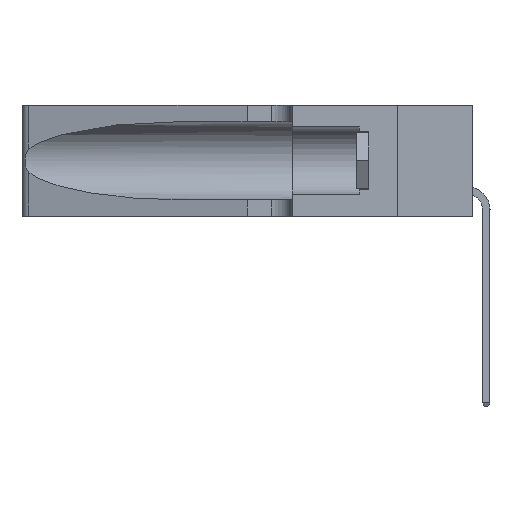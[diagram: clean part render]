
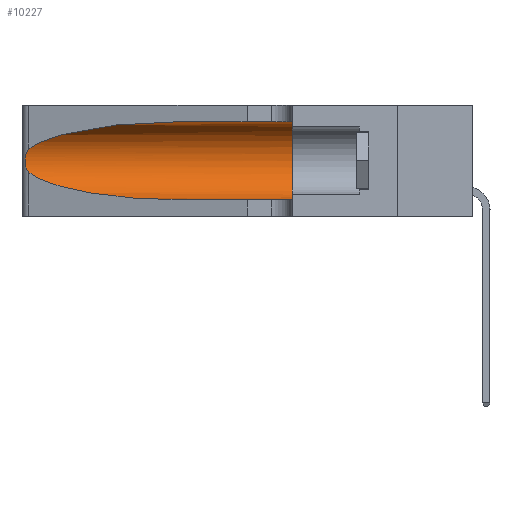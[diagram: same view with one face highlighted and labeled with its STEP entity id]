
A CAD part, left-side view. The second image highlights one B-rep face of the part: STEP entity #10227.
In plain terms, the highlighted cylindrical face has radius 3.308 mm (diameter 6.617 mm), a partial arc.
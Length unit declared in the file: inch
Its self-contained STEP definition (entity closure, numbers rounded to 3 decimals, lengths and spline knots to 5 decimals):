
#29 = DIRECTION ( 'NONE',  ( 0., -1., 0. ) ) ;
#494 = CARTESIAN_POINT ( 'NONE',  ( 0.25487, 1.22718, 0.14631 ) ) ;
#516 = DIRECTION ( 'NONE',  ( 0., 1., 0. ) ) ;
#2513 = CARTESIAN_POINT ( 'NONE',  ( 0.25487, 1.22718, 0.22369 ) ) ;
#2604 = CYLINDRICAL_SURFACE ( 'NONE', #42840, 0.13025 ) ;
#3637 = ORIENTED_EDGE ( 'NONE', *, *, #30311, .T. ) ;
#3889 = CARTESIAN_POINT ( 'NONE',  ( 0.18966, 0.96281, 0.31525 ) ) ;
#3982 = CARTESIAN_POINT ( 'NONE',  ( 0.1305, 0.35, 0.185 ) ) ;
#4868 = CARTESIAN_POINT ( 'NONE',  ( 0.1305, 0.72297, 0.05475 ) ) ;
#4972 = ORIENTED_EDGE ( 'NONE', *, *, #44741, .F. ) ;
#5165 = EDGE_CURVE ( 'NONE', #6816, #45733, #14179, .T. ) ;
#6179 = CARTESIAN_POINT ( 'NONE',  ( 0.1305, 0.72297, 0.05475 ) ) ;
#6353 = CARTESIAN_POINT ( 'NONE',  ( 0.25487, 1.22718, 0.22369 ) ) ;
#6499 = CARTESIAN_POINT ( 'NONE',  ( 0.2373, 1.15595, 0.08982 ) ) ;
#6816 = VERTEX_POINT ( 'NONE', #43045 ) ;
#7128 = DIRECTION ( 'NONE',  ( 0., -1., 0. ) ) ;
#7336 = CARTESIAN_POINT ( 'NONE',  ( 0.1305, 0.35, 0.31525 ) ) ;
#7553 = EDGE_CURVE ( 'NONE', #45733, #33437, #11917, .T. ) ;
#7561 = DIRECTION ( 'NONE',  ( 0., 0., 1. ) ) ;
#8125 = ORIENTED_EDGE ( 'NONE', *, *, #11375, .T. ) ;
#8598 = VERTEX_POINT ( 'NONE', #13550 ) ;
#10227 = ADVANCED_FACE ( 'NONE', ( #41705 ), #2604, .F. ) ;
#10822 = CARTESIAN_POINT ( 'NONE',  ( 0.25856, 1.23593, 0.16098 ) ) ;
#10857 = VECTOR ( 'NONE', #29, 39.37008 ) ;
#10958 = CARTESIAN_POINT ( 'NONE',  ( 0.26017, 1.23833, 0.17102 ) ) ;
#11375 = EDGE_CURVE ( 'NONE', #18134, #8598, #21839, .T. ) ;
#11917 = LINE ( 'NONE', #13009, #33744 ) ;
#12921 = VERTEX_POINT ( 'NONE', #7336 ) ;
#13009 = CARTESIAN_POINT ( 'NONE',  ( 0.1305, 1.61858, 0.05475 ) ) ;
#13550 = CARTESIAN_POINT ( 'NONE',  ( 0.25487, 1.22718, 0.22369 ) ) ;
#14179 =( BOUNDED_CURVE ( )  B_SPLINE_CURVE ( 3, ( #45401, #6499, #20214, #6179 ),
 .UNSPECIFIED., .F., .F. ) 
 B_SPLINE_CURVE_WITH_KNOTS ( ( 4, 4 ),
 ( 3.44316, 4.71239 ),
 .UNSPECIFIED. ) 
 CURVE ( )  GEOMETRIC_REPRESENTATION_ITEM ( )  RATIONAL_B_SPLINE_CURVE ( ( 1., 0.87, 0.87, 1. ) ) 
 REPRESENTATION_ITEM ( '' )  );
#14246 = ORIENTED_EDGE ( 'NONE', *, *, #33722, .F. ) ;
#14535 = CARTESIAN_POINT ( 'NONE',  ( 0.25639, 1.23186, 0.15144 ) ) ;
#14674 = CARTESIAN_POINT ( 'NONE',  ( 0.25854, 1.2359, 0.20912 ) ) ;
#15411 = CARTESIAN_POINT ( 'NONE',  ( 0.1305, 0.35, 0.05475 ) ) ;
#16484 = EDGE_LOOP ( 'NONE', ( #8125, #3637, #29158, #22478, #14246, #4972 ) ) ;
#17374 = CARTESIAN_POINT ( 'NONE',  ( 0.1305, 0.72297, 0.31525 ) ) ;
#17844 = CARTESIAN_POINT ( 'NONE',  ( 0.26075, 1.23896, 0.178 ) ) ;
#18134 = VERTEX_POINT ( 'NONE', #28069 ) ;
#20214 = CARTESIAN_POINT ( 'NONE',  ( 0.18966, 0.96281, 0.05475 ) ) ;
#20895 = CARTESIAN_POINT ( 'NONE',  ( 0.1305, 1.61858, 0.31525 ) ) ;
#21717 = CARTESIAN_POINT ( 'NONE',  ( 0.25555, 1.22994, 0.2215 ) ) ;
#21839 =( BOUNDED_CURVE ( )  B_SPLINE_CURVE ( 3, ( #17374, #3889, #29971, #2513 ),
 .UNSPECIFIED., .F., .F. ) 
 B_SPLINE_CURVE_WITH_KNOTS ( ( 4, 4 ),
 ( 1.5708, 2.84003 ),
 .UNSPECIFIED. ) 
 CURVE ( )  GEOMETRIC_REPRESENTATION_ITEM ( )  RATIONAL_B_SPLINE_CURVE ( ( 1., 0.87, 0.87, 1. ) ) 
 REPRESENTATION_ITEM ( '' )  );
#21869 = CARTESIAN_POINT ( 'NONE',  ( 0.25555, 1.22993, 0.14849 ) ) ;
#22018 = CARTESIAN_POINT ( 'NONE',  ( 0.25789, 1.23486, 0.15765 ) ) ;
#22478 = ORIENTED_EDGE ( 'NONE', *, *, #7553, .T. ) ;
#24600 = DIRECTION ( 'NONE',  ( 0., -1., 0. ) ) ;
#27795 = CARTESIAN_POINT ( 'NONE',  ( 0.1305, 1.61858, 0.185 ) ) ;
#28069 = CARTESIAN_POINT ( 'NONE',  ( 0.1305, 0.72297, 0.31525 ) ) ;
#29158 = ORIENTED_EDGE ( 'NONE', *, *, #5165, .T. ) ;
#29624 = B_SPLINE_CURVE_WITH_KNOTS ( 'NONE', 3,
 ( #6353, #21717, #35735, #39593, #14674, #32236, #39454, #17844, #10958, #10822, #22018, #14535, #21869, #494 ),
 .UNSPECIFIED., .F., .F.,
 ( 4, 2, 2, 2, 2, 2, 4 ),
 ( 0., 0.00027, 0.00053, 0.00107, 0.0016, 0.00187, 0.00214 ),
 .UNSPECIFIED. ) ;
#29971 = CARTESIAN_POINT ( 'NONE',  ( 0.2373, 1.15595, 0.28018 ) ) ;
#30311 = EDGE_CURVE ( 'NONE', #8598, #6816, #29624, .T. ) ;
#32236 = CARTESIAN_POINT ( 'NONE',  ( 0.26018, 1.23835, 0.19895 ) ) ;
#32290 = AXIS2_PLACEMENT_3D ( 'NONE', #3982, #516, #7561 ) ;
#33437 = VERTEX_POINT ( 'NONE', #15411 ) ;
#33722 = EDGE_CURVE ( 'NONE', #12921, #33437, #43496, .T. ) ;
#33744 = VECTOR ( 'NONE', #24600, 39.37008 ) ;
#35735 = CARTESIAN_POINT ( 'NONE',  ( 0.25639, 1.23184, 0.21858 ) ) ;
#35877 = DIRECTION ( 'NONE',  ( 0., 0., -1. ) ) ;
#36038 = LINE ( 'NONE', #20895, #10857 ) ;
#39454 = CARTESIAN_POINT ( 'NONE',  ( 0.26075, 1.23896, 0.19203 ) ) ;
#39593 = CARTESIAN_POINT ( 'NONE',  ( 0.25787, 1.23484, 0.2124 ) ) ;
#41705 = FACE_OUTER_BOUND ( 'NONE', #16484, .T. ) ;
#42840 = AXIS2_PLACEMENT_3D ( 'NONE', #27795, #7128, #35877 ) ;
#43045 = CARTESIAN_POINT ( 'NONE',  ( 0.25487, 1.22718, 0.14631 ) ) ;
#43496 = CIRCLE ( 'NONE', #32290, 0.13025 ) ;
#44741 = EDGE_CURVE ( 'NONE', #18134, #12921, #36038, .T. ) ;
#45401 = CARTESIAN_POINT ( 'NONE',  ( 0.25487, 1.22718, 0.14631 ) ) ;
#45733 = VERTEX_POINT ( 'NONE', #4868 ) ;
